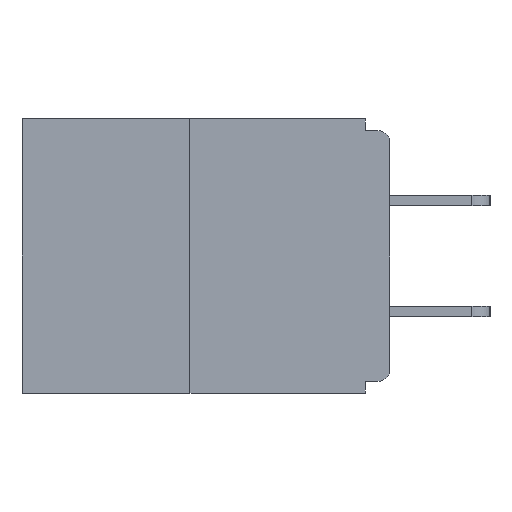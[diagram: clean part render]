
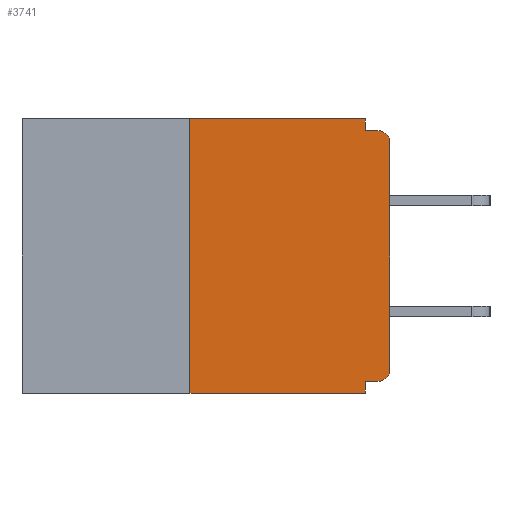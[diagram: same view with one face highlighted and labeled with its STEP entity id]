
A CAD part, left-side view. The second image highlights one B-rep face of the part: STEP entity #3741.
In plain terms, the highlighted planar face has unit normal (-1, 0, 0).
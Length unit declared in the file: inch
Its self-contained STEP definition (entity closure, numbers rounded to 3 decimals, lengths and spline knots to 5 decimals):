
#100 = DIRECTION ( 'NONE',  ( -1., 0., 0. ) ) ;
#246 = CARTESIAN_POINT ( 'NONE',  ( 0., 0.25, -0.343 ) ) ;
#357 = CARTESIAN_POINT ( 'NONE',  ( 0., 0.46, -0.343 ) ) ;
#468 = CARTESIAN_POINT ( 'NONE',  ( 0., 0., -0.03 ) ) ;
#489 = VECTOR ( 'NONE', #2791, 39.37008 ) ;
#775 = CARTESIAN_POINT ( 'NONE',  ( 0., 0., 0. ) ) ;
#841 = EDGE_CURVE ( 'NONE', #6232, #9821, #8862, .T. ) ;
#887 = VECTOR ( 'NONE', #5698, 39.37008 ) ;
#998 = EDGE_CURVE ( 'NONE', #11899, #6119, #8358, .T. ) ;
#1474 = CARTESIAN_POINT ( 'NONE',  ( 0., 0.015, -0.03 ) ) ;
#1539 = CARTESIAN_POINT ( 'NONE',  ( 0., 0.031, -0.328 ) ) ;
#1811 = EDGE_CURVE ( 'NONE', #12605, #6232, #10321, .T. ) ;
#1940 = EDGE_CURVE ( 'NONE', #11263, #12605, #6305, .T. ) ;
#2022 = DIRECTION ( 'NONE',  ( 0., 0., -1. ) ) ;
#2157 = EDGE_CURVE ( 'NONE', #11899, #11263, #16722, .T. ) ;
#2758 = EDGE_LOOP ( 'NONE', ( #6722, #16700, #3085, #18557, #7710, #16577, #3130, #18089, #17954, #11094 ) ) ;
#2791 = DIRECTION ( 'NONE',  ( 0., 0., -1. ) ) ;
#2808 = CIRCLE ( 'NONE', #12895, 0.015 ) ;
#3039 = DIRECTION ( 'NONE',  ( 0., -1., 0. ) ) ;
#3066 = CARTESIAN_POINT ( 'NONE',  ( 0., 0.031, -0.015 ) ) ;
#3085 = ORIENTED_EDGE ( 'NONE', *, *, #998, .T. ) ;
#3130 = ORIENTED_EDGE ( 'NONE', *, *, #20609, .T. ) ;
#3352 = EDGE_CURVE ( 'NONE', #13105, #6119, #4385, .T. ) ;
#3594 = VECTOR ( 'NONE', #3039, 39.37008 ) ;
#3741 = ADVANCED_FACE ( 'NONE', ( #8993 ), #4249, .F. ) ;
#4249 = PLANE ( 'NONE',  #14962 ) ;
#4385 = LINE ( 'NONE', #17240, #489 ) ;
#4567 = DIRECTION ( 'NONE',  ( 1., 0., 0. ) ) ;
#4643 = VECTOR ( 'NONE', #13089, 39.37008 ) ;
#5317 = DIRECTION ( 'NONE',  ( 0., 0., 1. ) ) ;
#5698 = DIRECTION ( 'NONE',  ( 0., 0., -1. ) ) ;
#6119 = VERTEX_POINT ( 'NONE', #15388 ) ;
#6232 = VERTEX_POINT ( 'NONE', #3066 ) ;
#6305 = LINE ( 'NONE', #14097, #3594 ) ;
#6722 = ORIENTED_EDGE ( 'NONE', *, *, #1940, .F. ) ;
#6767 = VECTOR ( 'NONE', #16442, 39.37008 ) ;
#7397 = CARTESIAN_POINT ( 'NONE',  ( 0., 0.031, 0. ) ) ;
#7710 = ORIENTED_EDGE ( 'NONE', *, *, #12481, .F. ) ;
#7839 = DIRECTION ( 'NONE',  ( 0., 0., -1. ) ) ;
#8001 = CARTESIAN_POINT ( 'NONE',  ( 0., 0.015, -0.015 ) ) ;
#8358 = LINE ( 'NONE', #357, #4643 ) ;
#8451 = CARTESIAN_POINT ( 'NONE',  ( 0., 0.015, -0.328 ) ) ;
#8862 = LINE ( 'NONE', #10439, #19152 ) ;
#8993 = FACE_OUTER_BOUND ( 'NONE', #2758, .T. ) ;
#9821 = VERTEX_POINT ( 'NONE', #8001 ) ;
#10321 = LINE ( 'NONE', #16644, #887 ) ;
#10439 = CARTESIAN_POINT ( 'NONE',  ( 0., 0., -0.015 ) ) ;
#11094 = ORIENTED_EDGE ( 'NONE', *, *, #1811, .F. ) ;
#11263 = VERTEX_POINT ( 'NONE', #16654 ) ;
#11516 = CARTESIAN_POINT ( 'NONE',  ( 0., 0.015, -0.313 ) ) ;
#11899 = VERTEX_POINT ( 'NONE', #246 ) ;
#12481 = EDGE_CURVE ( 'NONE', #17957, #13105, #14868, .T. ) ;
#12605 = VERTEX_POINT ( 'NONE', #7397 ) ;
#12895 = AXIS2_PLACEMENT_3D ( 'NONE', #1474, #100, #14631 ) ;
#13089 = DIRECTION ( 'NONE',  ( 0., -1., 0. ) ) ;
#13105 = VERTEX_POINT ( 'NONE', #1539 ) ;
#13390 = DIRECTION ( 'NONE',  ( 0., -1., 0. ) ) ;
#13404 = EDGE_CURVE ( 'NONE', #20434, #9821, #2808, .T. ) ;
#13723 = LINE ( 'NONE', #775, #17857 ) ;
#14097 = CARTESIAN_POINT ( 'NONE',  ( 0., 0.46, 0. ) ) ;
#14338 = AXIS2_PLACEMENT_3D ( 'NONE', #11516, #16448, #2022 ) ;
#14631 = DIRECTION ( 'NONE',  ( 0., 0., -1. ) ) ;
#14868 = LINE ( 'NONE', #14972, #6767 ) ;
#14962 = AXIS2_PLACEMENT_3D ( 'NONE', #19002, #4567, #7839 ) ;
#14972 = CARTESIAN_POINT ( 'NONE',  ( 0., 0., -0.328 ) ) ;
#15139 = CARTESIAN_POINT ( 'NONE',  ( 0., 0.25, 0. ) ) ;
#15388 = CARTESIAN_POINT ( 'NONE',  ( 0., 0.031, -0.343 ) ) ;
#16247 = EDGE_CURVE ( 'NONE', #17957, #19231, #17053, .T. ) ;
#16442 = DIRECTION ( 'NONE',  ( 0., 1., 0. ) ) ;
#16448 = DIRECTION ( 'NONE',  ( -1., 0., 0. ) ) ;
#16577 = ORIENTED_EDGE ( 'NONE', *, *, #16247, .T. ) ;
#16644 = CARTESIAN_POINT ( 'NONE',  ( 0., 0.031, 0. ) ) ;
#16654 = CARTESIAN_POINT ( 'NONE',  ( 0., 0.25, 0. ) ) ;
#16700 = ORIENTED_EDGE ( 'NONE', *, *, #2157, .F. ) ;
#16722 = LINE ( 'NONE', #15139, #20097 ) ;
#17053 = CIRCLE ( 'NONE', #14338, 0.015 ) ;
#17240 = CARTESIAN_POINT ( 'NONE',  ( 0., 0.031, -0.343 ) ) ;
#17857 = VECTOR ( 'NONE', #5317, 39.37008 ) ;
#17954 = ORIENTED_EDGE ( 'NONE', *, *, #841, .F. ) ;
#17957 = VERTEX_POINT ( 'NONE', #8451 ) ;
#18089 = ORIENTED_EDGE ( 'NONE', *, *, #13404, .T. ) ;
#18213 = DIRECTION ( 'NONE',  ( 0., 0., 1. ) ) ;
#18257 = CARTESIAN_POINT ( 'NONE',  ( 0., 0., -0.313 ) ) ;
#18557 = ORIENTED_EDGE ( 'NONE', *, *, #3352, .F. ) ;
#19002 = CARTESIAN_POINT ( 'NONE',  ( 0., 0.46, 0. ) ) ;
#19152 = VECTOR ( 'NONE', #13390, 39.37008 ) ;
#19231 = VERTEX_POINT ( 'NONE', #18257 ) ;
#20097 = VECTOR ( 'NONE', #18213, 39.37008 ) ;
#20434 = VERTEX_POINT ( 'NONE', #468 ) ;
#20609 = EDGE_CURVE ( 'NONE', #19231, #20434, #13723, .T. ) ;
